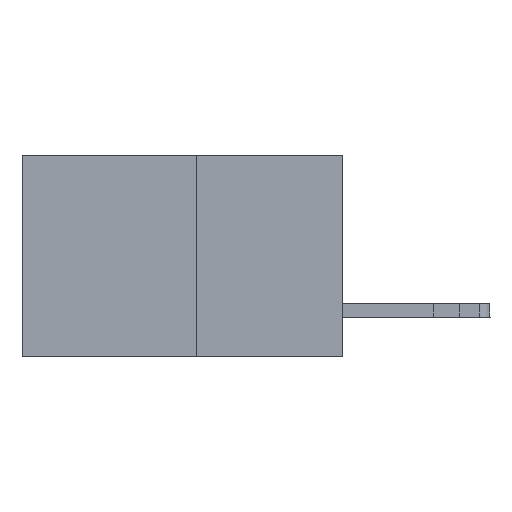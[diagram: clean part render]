
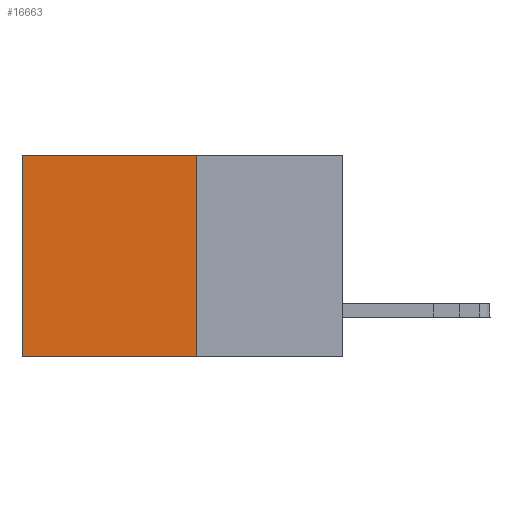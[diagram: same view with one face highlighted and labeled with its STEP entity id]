
A CAD part, left-side view. The second image highlights one B-rep face of the part: STEP entity #16663.
In plain terms, the highlighted planar face has unit normal (-1, 0, 0).
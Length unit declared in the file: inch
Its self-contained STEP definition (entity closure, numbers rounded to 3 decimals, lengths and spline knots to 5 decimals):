
#301 = CARTESIAN_POINT ( 'NONE',  ( 0.277, 0.27, -0.37 ) ) ;
#798 = FACE_OUTER_BOUND ( 'NONE', #1868, .T. ) ;
#1210 = CARTESIAN_POINT ( 'NONE',  ( 0.277, 0.59, 0. ) ) ;
#1868 = EDGE_LOOP ( 'NONE', ( #23898, #7349, #5380, #16643 ) ) ;
#2880 = LINE ( 'NONE', #12608, #8472 ) ;
#3038 = DIRECTION ( 'NONE',  ( 0., 1., 0. ) ) ;
#5380 = ORIENTED_EDGE ( 'NONE', *, *, #30323, .F. ) ;
#7349 = ORIENTED_EDGE ( 'NONE', *, *, #20455, .F. ) ;
#7356 = CARTESIAN_POINT ( 'NONE',  ( 0.277, 0.59, -0.37 ) ) ;
#8137 = DIRECTION ( 'NONE',  ( 1., 0., 0. ) ) ;
#8356 = VECTOR ( 'NONE', #12121, 39.37008 ) ;
#8472 = VECTOR ( 'NONE', #3038, 39.37008 ) ;
#9951 = EDGE_CURVE ( 'NONE', #15141, #10356, #2880, .T. ) ;
#10356 = VERTEX_POINT ( 'NONE', #1210 ) ;
#12121 = DIRECTION ( 'NONE',  ( 0., 0., -1. ) ) ;
#12608 = CARTESIAN_POINT ( 'NONE',  ( 0.277, 0.27, 0. ) ) ;
#13272 = VECTOR ( 'NONE', #27551, 39.37008 ) ;
#14096 = CARTESIAN_POINT ( 'NONE',  ( 0.277, 0.59, -0.37 ) ) ;
#14873 = EDGE_CURVE ( 'NONE', #10356, #22643, #29175, .T. ) ;
#15141 = VERTEX_POINT ( 'NONE', #25228 ) ;
#15156 = DIRECTION ( 'NONE',  ( 0., 0., -1. ) ) ;
#15226 = AXIS2_PLACEMENT_3D ( 'NONE', #27256, #8137, #15156 ) ;
#16539 = CARTESIAN_POINT ( 'NONE',  ( 0.277, 0.27, -0.37 ) ) ;
#16643 = ORIENTED_EDGE ( 'NONE', *, *, #9951, .T. ) ;
#16663 = ADVANCED_FACE ( 'NONE', ( #798 ), #25196, .F. ) ;
#18543 = VERTEX_POINT ( 'NONE', #27782 ) ;
#18779 = LINE ( 'NONE', #16539, #26548 ) ;
#20455 = EDGE_CURVE ( 'NONE', #18543, #22643, #18779, .T. ) ;
#22145 = LINE ( 'NONE', #301, #13272 ) ;
#22643 = VERTEX_POINT ( 'NONE', #14096 ) ;
#23898 = ORIENTED_EDGE ( 'NONE', *, *, #14873, .T. ) ;
#25196 = PLANE ( 'NONE',  #15226 ) ;
#25228 = CARTESIAN_POINT ( 'NONE',  ( 0.277, 0.27, 0. ) ) ;
#26548 = VECTOR ( 'NONE', #28491, 39.37008 ) ;
#27256 = CARTESIAN_POINT ( 'NONE',  ( 0.277, 0.27, -0.37 ) ) ;
#27551 = DIRECTION ( 'NONE',  ( 0., 0., -1. ) ) ;
#27782 = CARTESIAN_POINT ( 'NONE',  ( 0.277, 0.27, -0.37 ) ) ;
#28491 = DIRECTION ( 'NONE',  ( 0., 1., 0. ) ) ;
#29175 = LINE ( 'NONE', #7356, #8356 ) ;
#30323 = EDGE_CURVE ( 'NONE', #15141, #18543, #22145, .T. ) ;
